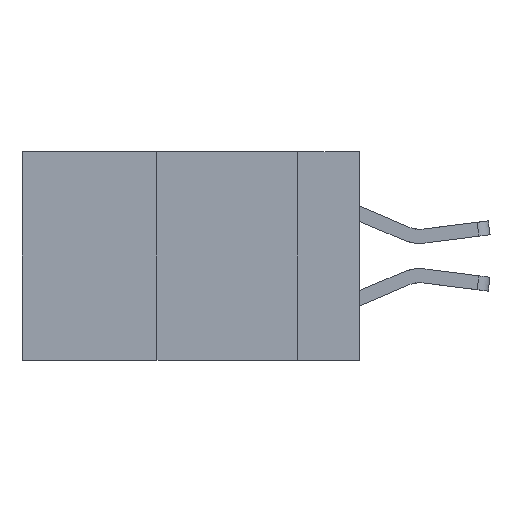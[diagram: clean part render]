
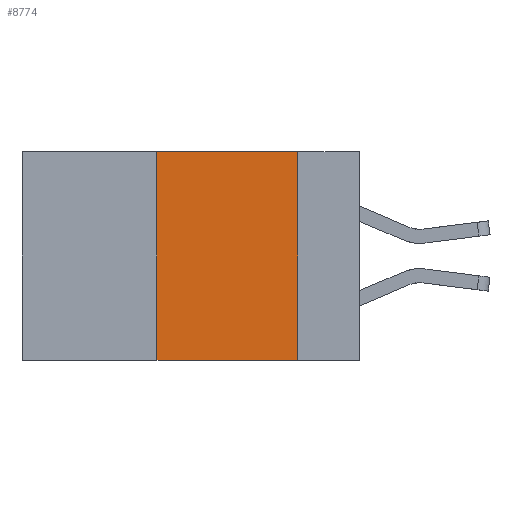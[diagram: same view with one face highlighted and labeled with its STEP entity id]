
A CAD part, left-side view. The second image highlights one B-rep face of the part: STEP entity #8774.
In plain terms, the highlighted planar face has unit normal (-1, 0, 0).
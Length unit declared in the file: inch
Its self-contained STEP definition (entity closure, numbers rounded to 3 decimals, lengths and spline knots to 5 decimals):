
#10 = VECTOR ( 'NONE', #3388, 39.37008 ) ;
#119 = LINE ( 'NONE', #1099, #10 ) ;
#385 = CARTESIAN_POINT ( 'NONE',  ( 0., 0.36, 0. ) ) ;
#1005 = ORIENTED_EDGE ( 'NONE', *, *, #1530, .F. ) ;
#1099 = CARTESIAN_POINT ( 'NONE',  ( 0., 0.6, 0. ) ) ;
#1212 = LINE ( 'NONE', #9302, #7858 ) ;
#1530 = EDGE_CURVE ( 'NONE', #4625, #9756, #6652, .T. ) ;
#1617 = VECTOR ( 'NONE', #9676, 39.37008 ) ;
#1803 = CARTESIAN_POINT ( 'NONE',  ( 0., 0.36, 0. ) ) ;
#1818 = VERTEX_POINT ( 'NONE', #7752 ) ;
#2395 = PLANE ( 'NONE',  #4988 ) ;
#3064 = ORIENTED_EDGE ( 'NONE', *, *, #6721, .F. ) ;
#3108 = LINE ( 'NONE', #5867, #1617 ) ;
#3110 = DIRECTION ( 'NONE',  ( 0., 0., -1. ) ) ;
#3388 = DIRECTION ( 'NONE',  ( 0., -1., 0. ) ) ;
#3926 = DIRECTION ( 'NONE',  ( 1., 0., 0. ) ) ;
#4095 = VECTOR ( 'NONE', #6587, 39.37008 ) ;
#4625 = VERTEX_POINT ( 'NONE', #5880 ) ;
#4988 = AXIS2_PLACEMENT_3D ( 'NONE', #7782, #3926, #3110 ) ;
#5362 = DIRECTION ( 'NONE',  ( 0., 0., -1. ) ) ;
#5867 = CARTESIAN_POINT ( 'NONE',  ( 0., 0.6, -0.37 ) ) ;
#5880 = CARTESIAN_POINT ( 'NONE',  ( 0., 0.36, -0.37 ) ) ;
#5891 = EDGE_CURVE ( 'NONE', #9756, #7977, #119, .T. ) ;
#6233 = EDGE_LOOP ( 'NONE', ( #3064, #7082, #1005, #8383 ) ) ;
#6587 = DIRECTION ( 'NONE',  ( 0., 0., 1. ) ) ;
#6652 = LINE ( 'NONE', #385, #4095 ) ;
#6721 = EDGE_CURVE ( 'NONE', #7977, #1818, #1212, .T. ) ;
#7082 = ORIENTED_EDGE ( 'NONE', *, *, #5891, .F. ) ;
#7515 = CARTESIAN_POINT ( 'NONE',  ( 0., 0.11, 0. ) ) ;
#7752 = CARTESIAN_POINT ( 'NONE',  ( 0., 0.11, -0.37 ) ) ;
#7782 = CARTESIAN_POINT ( 'NONE',  ( 0., 0.6, 0. ) ) ;
#7858 = VECTOR ( 'NONE', #5362, 39.37008 ) ;
#7977 = VERTEX_POINT ( 'NONE', #7515 ) ;
#8383 = ORIENTED_EDGE ( 'NONE', *, *, #8499, .T. ) ;
#8499 = EDGE_CURVE ( 'NONE', #4625, #1818, #3108, .T. ) ;
#8774 = ADVANCED_FACE ( 'NONE', ( #9978 ), #2395, .F. ) ;
#9302 = CARTESIAN_POINT ( 'NONE',  ( 0., 0.11, 0. ) ) ;
#9676 = DIRECTION ( 'NONE',  ( 0., -1., 0. ) ) ;
#9756 = VERTEX_POINT ( 'NONE', #1803 ) ;
#9978 = FACE_OUTER_BOUND ( 'NONE', #6233, .T. ) ;
